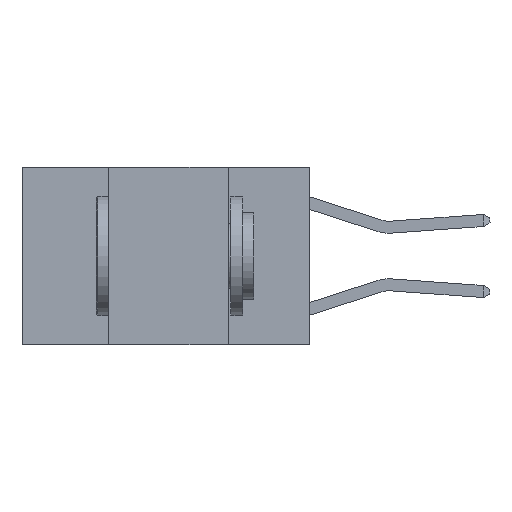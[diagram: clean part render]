
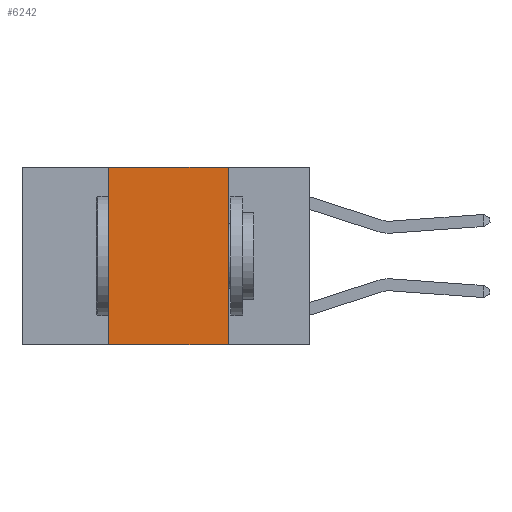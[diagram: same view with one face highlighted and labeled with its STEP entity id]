
A CAD part, left-side view. The second image highlights one B-rep face of the part: STEP entity #6242.
In plain terms, the highlighted planar face has unit normal (-1, 0, 0).
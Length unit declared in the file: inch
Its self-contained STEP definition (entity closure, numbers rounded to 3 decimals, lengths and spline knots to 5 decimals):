
#78 = VERTEX_POINT ( 'NONE', #11544 ) ;
#1328 = CARTESIAN_POINT ( 'NONE',  ( 0., 0.42, -0.37 ) ) ;
#1642 = ORIENTED_EDGE ( 'NONE', *, *, #16333, .F. ) ;
#2262 = VECTOR ( 'NONE', #15988, 39.37008 ) ;
#2388 = EDGE_CURVE ( 'NONE', #3291, #13100, #7890, .T. ) ;
#3065 = CARTESIAN_POINT ( 'NONE',  ( 0., 0.17, 0. ) ) ;
#3291 = VERTEX_POINT ( 'NONE', #1328 ) ;
#3362 = VERTEX_POINT ( 'NONE', #3065 ) ;
#4472 = DIRECTION ( 'NONE',  ( 0., 0., -1. ) ) ;
#6242 = ADVANCED_FACE ( 'NONE', ( #9261 ), #19774, .F. ) ;
#7890 = LINE ( 'NONE', #10344, #19099 ) ;
#9261 = FACE_OUTER_BOUND ( 'NONE', #19748, .T. ) ;
#10049 = ORIENTED_EDGE ( 'NONE', *, *, #2388, .T. ) ;
#10190 = EDGE_CURVE ( 'NONE', #3362, #13100, #14723, .T. ) ;
#10269 = DIRECTION ( 'NONE',  ( 0., -1., 0. ) ) ;
#10344 = CARTESIAN_POINT ( 'NONE',  ( 0., 0.6, -0.37 ) ) ;
#10761 = CARTESIAN_POINT ( 'NONE',  ( 0., 0.6, 0. ) ) ;
#11544 = CARTESIAN_POINT ( 'NONE',  ( 0., 0.42, 0. ) ) ;
#12699 = ORIENTED_EDGE ( 'NONE', *, *, #10190, .F. ) ;
#13014 = VECTOR ( 'NONE', #14317, 39.37008 ) ;
#13100 = VERTEX_POINT ( 'NONE', #17189 ) ;
#13196 = ORIENTED_EDGE ( 'NONE', *, *, #16702, .F. ) ;
#13835 = DIRECTION ( 'NONE',  ( 1., 0., 0. ) ) ;
#13984 = LINE ( 'NONE', #15759, #13014 ) ;
#14317 = DIRECTION ( 'NONE',  ( 0., 0., 1. ) ) ;
#14417 = LINE ( 'NONE', #19591, #17923 ) ;
#14493 = CARTESIAN_POINT ( 'NONE',  ( 0., 0.17, 0. ) ) ;
#14723 = LINE ( 'NONE', #14493, #2262 ) ;
#15759 = CARTESIAN_POINT ( 'NONE',  ( 0., 0.42, 0. ) ) ;
#15988 = DIRECTION ( 'NONE',  ( 0., 0., -1. ) ) ;
#16333 = EDGE_CURVE ( 'NONE', #3291, #78, #13984, .T. ) ;
#16621 = AXIS2_PLACEMENT_3D ( 'NONE', #10761, #13835, #4472 ) ;
#16702 = EDGE_CURVE ( 'NONE', #78, #3362, #14417, .T. ) ;
#17189 = CARTESIAN_POINT ( 'NONE',  ( 0., 0.17, -0.37 ) ) ;
#17923 = VECTOR ( 'NONE', #18089, 39.37008 ) ;
#18089 = DIRECTION ( 'NONE',  ( 0., -1., 0. ) ) ;
#19099 = VECTOR ( 'NONE', #10269, 39.37008 ) ;
#19591 = CARTESIAN_POINT ( 'NONE',  ( 0., 0.6, 0. ) ) ;
#19748 = EDGE_LOOP ( 'NONE', ( #12699, #13196, #1642, #10049 ) ) ;
#19774 = PLANE ( 'NONE',  #16621 ) ;
